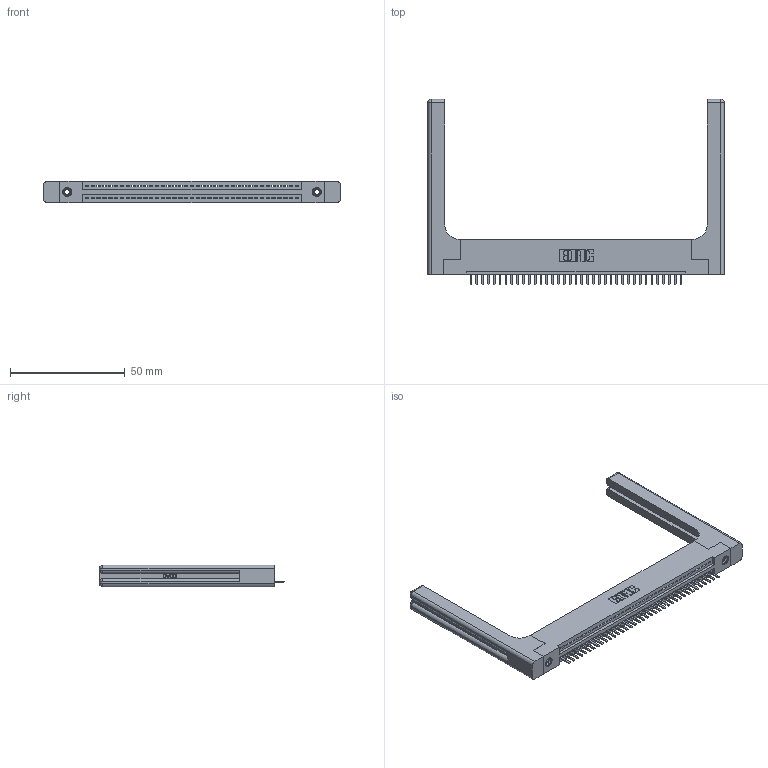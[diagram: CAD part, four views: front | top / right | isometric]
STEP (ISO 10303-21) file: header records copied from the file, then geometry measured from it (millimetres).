
FILE_DESCRIPTION (( 'STEP AP203' ), '1' );
FILE_NAME ('395-037-520-158.STEP', '2019-10-21T22:46:18', ( '' ), ( '' ), 'SwSTEP 2.0', 'SolidWorks 2016', '' );
FILE_SCHEMA (( 'CONFIG_CONTROL_DESIGN' ));
Length unit declared in the file: inch
Products named in the file (5): 345 Part_Flush Mounting Lugs - 0.156 Dia-TH; 345-292-001_345-293-120; 395-037-520-158; 345-220-058_345-220-058; 345-250-001_345-250-001-102
Assembly tree (42 placements, depth 2):
  395-037-520-158
    345 Part_Flush Mounting Lugs - 0.156 Dia-TH
    345-292-001_345-293-120  x37
    345-250-001_345-250-001-102  x2
    345-220-058_345-220-058  x2
Bounding box: 129.01 x 80.64 x 9.4 mm (x, y, z)
Volume: 20610.7 mm3; surface area: 20976.9 mm2
Topology: 42 solids, 42 shells, 2676 faces, 7815 edges, 5090 vertices
Faces by surface type: plane 1782, cylinder 834, bspline 36, cone 12, sphere 8, torus 4
Entity records: 33816 total; most frequent: CARTESIAN_POINT 6840, ORIENTED_EDGE 5596, DIRECTION 4916, EDGE_CURVE 2798, LINE 2422, VECTOR 2422, VERTEX_POINT 1854, AXIS2_PLACEMENT_3D 1247
